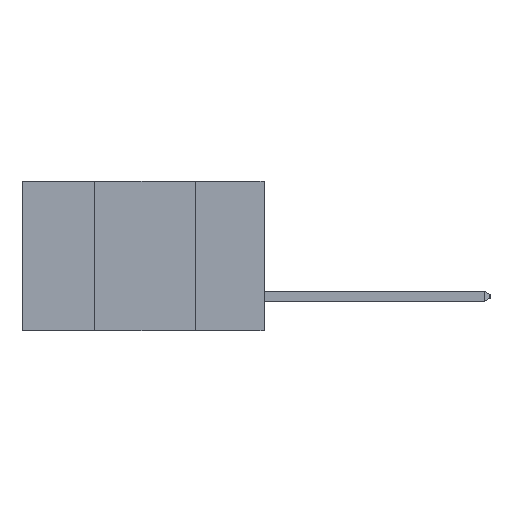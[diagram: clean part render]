
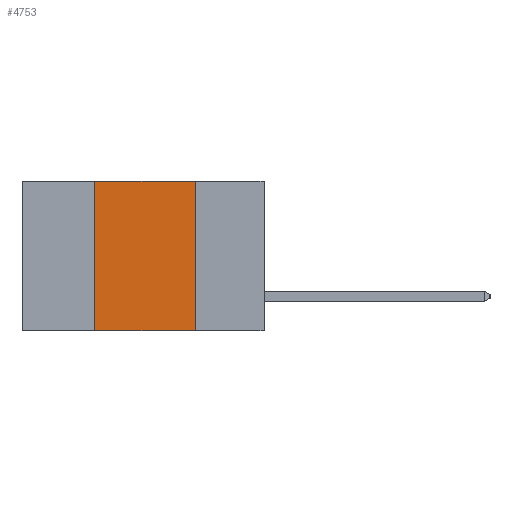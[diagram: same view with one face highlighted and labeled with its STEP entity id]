
A CAD part, left-side view. The second image highlights one B-rep face of the part: STEP entity #4753.
In plain terms, the highlighted planar face has unit normal (-1, 0, 0).
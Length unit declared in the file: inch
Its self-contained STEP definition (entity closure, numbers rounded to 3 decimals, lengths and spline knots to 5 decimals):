
#2631 = EDGE_CURVE ( 'NONE', #6711, #21170, #2959, .T. ) ;
#2920 = EDGE_CURVE ( 'NONE', #14735, #21170, #12580, .T. ) ;
#2959 = LINE ( 'NONE', #6338, #14418 ) ;
#4021 = VECTOR ( 'NONE', #16906, 39.37008 ) ;
#4753 = ADVANCED_FACE ( 'NONE', ( #11186 ), #5919, .F. ) ;
#5102 = ORIENTED_EDGE ( 'NONE', *, *, #2920, .T. ) ;
#5683 = EDGE_CURVE ( 'NONE', #12666, #6711, #15044, .T. ) ;
#5844 = DIRECTION ( 'NONE',  ( 0., 0., -1. ) ) ;
#5872 = DIRECTION ( 'NONE',  ( 1., 0., 0. ) ) ;
#5919 = PLANE ( 'NONE',  #8746 ) ;
#6002 = DIRECTION ( 'NONE',  ( 0., 0., -1. ) ) ;
#6064 = CARTESIAN_POINT ( 'NONE',  ( 0., 0.6, 0. ) ) ;
#6338 = CARTESIAN_POINT ( 'NONE',  ( 0., 0.17, -0.37 ) ) ;
#6711 = VERTEX_POINT ( 'NONE', #22103 ) ;
#8364 = CARTESIAN_POINT ( 'NONE',  ( 0., 0.42, 0. ) ) ;
#8746 = AXIS2_PLACEMENT_3D ( 'NONE', #6064, #5872, #5844 ) ;
#10072 = VECTOR ( 'NONE', #16830, 39.37008 ) ;
#11186 = FACE_OUTER_BOUND ( 'NONE', #14633, .T. ) ;
#11825 = DIRECTION ( 'NONE',  ( 0., 0., 1. ) ) ;
#12580 = LINE ( 'NONE', #17042, #4021 ) ;
#12666 = VERTEX_POINT ( 'NONE', #8364 ) ;
#12756 = CARTESIAN_POINT ( 'NONE',  ( 0., 0.42, -0.37 ) ) ;
#13319 = CARTESIAN_POINT ( 'NONE',  ( 0., 0.17, -0.37 ) ) ;
#14418 = VECTOR ( 'NONE', #6002, 39.37008 ) ;
#14633 = EDGE_LOOP ( 'NONE', ( #21309, #20175, #19501, #5102 ) ) ;
#14735 = VERTEX_POINT ( 'NONE', #12756 ) ;
#15044 = LINE ( 'NONE', #16787, #10072 ) ;
#16634 = LINE ( 'NONE', #21990, #20752 ) ;
#16787 = CARTESIAN_POINT ( 'NONE',  ( 0., 0.6, 0. ) ) ;
#16830 = DIRECTION ( 'NONE',  ( 0., -1., 0. ) ) ;
#16906 = DIRECTION ( 'NONE',  ( 0., -1., 0. ) ) ;
#17042 = CARTESIAN_POINT ( 'NONE',  ( 0., 0.6, -0.37 ) ) ;
#19501 = ORIENTED_EDGE ( 'NONE', *, *, #20564, .F. ) ;
#20175 = ORIENTED_EDGE ( 'NONE', *, *, #5683, .F. ) ;
#20564 = EDGE_CURVE ( 'NONE', #14735, #12666, #16634, .T. ) ;
#20752 = VECTOR ( 'NONE', #11825, 39.37008 ) ;
#21170 = VERTEX_POINT ( 'NONE', #13319 ) ;
#21309 = ORIENTED_EDGE ( 'NONE', *, *, #2631, .F. ) ;
#21990 = CARTESIAN_POINT ( 'NONE',  ( 0., 0.42, -0.37 ) ) ;
#22103 = CARTESIAN_POINT ( 'NONE',  ( 0., 0.17, 0. ) ) ;
